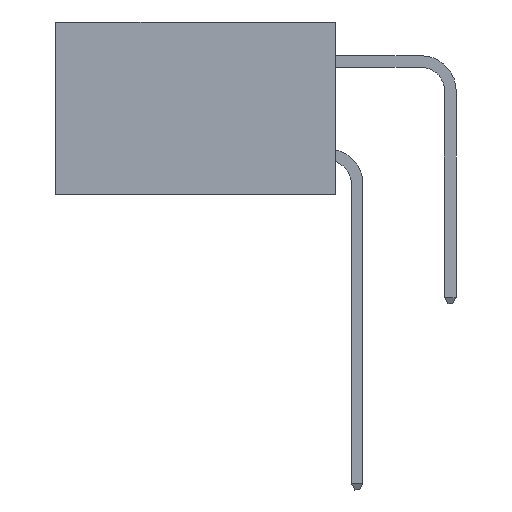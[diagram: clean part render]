
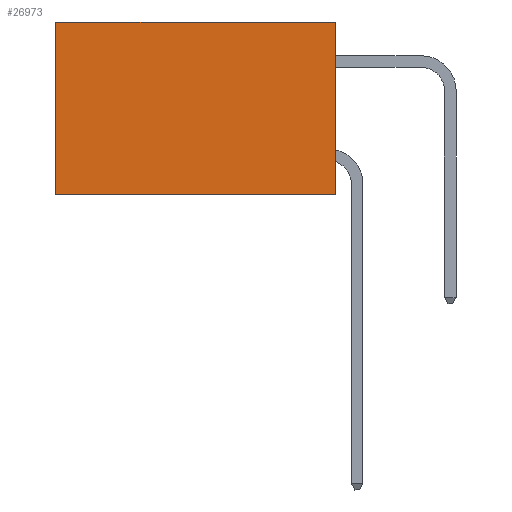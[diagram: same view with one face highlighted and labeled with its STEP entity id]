
A CAD part, left-side view. The second image highlights one B-rep face of the part: STEP entity #26973.
In plain terms, the highlighted planar face has unit normal (-1, 0, 0).
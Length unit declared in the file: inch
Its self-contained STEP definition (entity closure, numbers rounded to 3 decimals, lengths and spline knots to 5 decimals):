
#913 = EDGE_CURVE ( 'NONE', #7524, #25046, #24078, .T. ) ;
#4129 = PLANE ( 'NONE',  #16704 ) ;
#4363 = CARTESIAN_POINT ( 'NONE',  ( 0.2875, 0., 0. ) ) ;
#5545 = EDGE_CURVE ( 'NONE', #14912, #7524, #25872, .T. ) ;
#7345 = CARTESIAN_POINT ( 'NONE',  ( 0.2875, 0., -0.37 ) ) ;
#7524 = VERTEX_POINT ( 'NONE', #7345 ) ;
#7595 = CARTESIAN_POINT ( 'NONE',  ( 0.2875, 0., 0. ) ) ;
#8487 = ORIENTED_EDGE ( 'NONE', *, *, #31682, .T. ) ;
#9985 = DIRECTION ( 'NONE',  ( 1., 0., 0. ) ) ;
#12820 = DIRECTION ( 'NONE',  ( 0., 0., -1. ) ) ;
#13606 = EDGE_LOOP ( 'NONE', ( #8487, #16955, #32439, #20440 ) ) ;
#13964 = DIRECTION ( 'NONE',  ( 0., 0., -1. ) ) ;
#14912 = VERTEX_POINT ( 'NONE', #35294 ) ;
#15735 = LINE ( 'NONE', #7595, #19678 ) ;
#16704 = AXIS2_PLACEMENT_3D ( 'NONE', #4363, #9985, #12820 ) ;
#16955 = ORIENTED_EDGE ( 'NONE', *, *, #913, .F. ) ;
#18905 = CARTESIAN_POINT ( 'NONE',  ( 0.2875, 0.6, -0.37 ) ) ;
#19678 = VECTOR ( 'NONE', #32864, 39.37008 ) ;
#19728 = VECTOR ( 'NONE', #34011, 39.37008 ) ;
#20440 = ORIENTED_EDGE ( 'NONE', *, *, #31185, .T. ) ;
#21560 = VERTEX_POINT ( 'NONE', #32885 ) ;
#22800 = CARTESIAN_POINT ( 'NONE',  ( 0.2875, 0., -0.37 ) ) ;
#23195 = VECTOR ( 'NONE', #34083, 39.37008 ) ;
#24078 = LINE ( 'NONE', #22800, #23195 ) ;
#25046 = VERTEX_POINT ( 'NONE', #18905 ) ;
#25872 = LINE ( 'NONE', #28139, #19728 ) ;
#26973 = ADVANCED_FACE ( 'NONE', ( #34476 ), #4129, .F. ) ;
#27945 = CARTESIAN_POINT ( 'NONE',  ( 0.2875, 0.6, 0. ) ) ;
#28139 = CARTESIAN_POINT ( 'NONE',  ( 0.2875, 0., 0. ) ) ;
#31185 = EDGE_CURVE ( 'NONE', #14912, #21560, #15735, .T. ) ;
#31682 = EDGE_CURVE ( 'NONE', #21560, #25046, #35853, .T. ) ;
#32322 = VECTOR ( 'NONE', #13964, 39.37008 ) ;
#32439 = ORIENTED_EDGE ( 'NONE', *, *, #5545, .F. ) ;
#32864 = DIRECTION ( 'NONE',  ( 0., 1., 0. ) ) ;
#32885 = CARTESIAN_POINT ( 'NONE',  ( 0.2875, 0.6, 0. ) ) ;
#34011 = DIRECTION ( 'NONE',  ( 0., 0., -1. ) ) ;
#34083 = DIRECTION ( 'NONE',  ( 0., 1., 0. ) ) ;
#34476 = FACE_OUTER_BOUND ( 'NONE', #13606, .T. ) ;
#35294 = CARTESIAN_POINT ( 'NONE',  ( 0.2875, 0., 0. ) ) ;
#35853 = LINE ( 'NONE', #27945, #32322 ) ;
